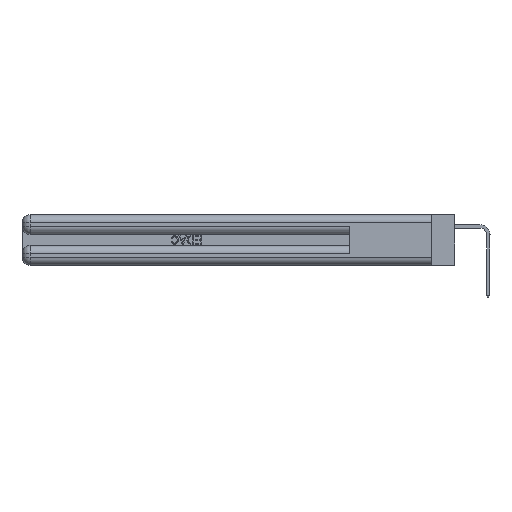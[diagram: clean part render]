
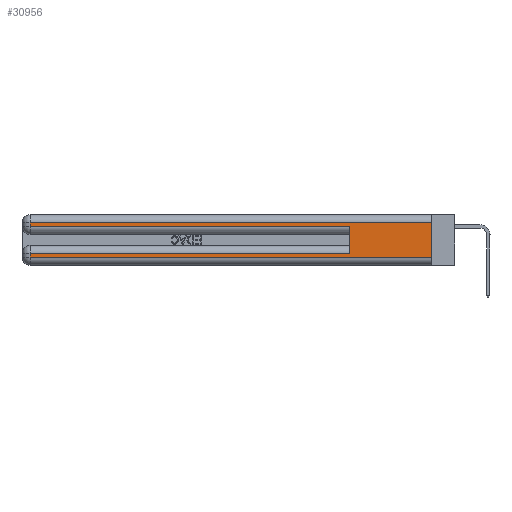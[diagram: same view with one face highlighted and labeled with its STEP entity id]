
A CAD part, left-side view. The second image highlights one B-rep face of the part: STEP entity #30956.
In plain terms, the highlighted planar face has unit normal (-1, 0, 0).
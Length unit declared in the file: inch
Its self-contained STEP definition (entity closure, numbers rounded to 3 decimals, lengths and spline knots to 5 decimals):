
#884 = CARTESIAN_POINT ( 'NONE',  ( 0., 2.94, 0.37 ) ) ;
#974 = VERTEX_POINT ( 'NONE', #17240 ) ;
#1247 = VECTOR ( 'NONE', #31002, 39.37008 ) ;
#1819 = VECTOR ( 'NONE', #13228, 39.37008 ) ;
#2746 = CARTESIAN_POINT ( 'NONE',  ( 0., 2.94, 0.37 ) ) ;
#3837 = VERTEX_POINT ( 'NONE', #28494 ) ;
#3931 = VERTEX_POINT ( 'NONE', #13141 ) ;
#4986 = CARTESIAN_POINT ( 'NONE',  ( 0., 0., 0.06 ) ) ;
#6003 = EDGE_CURVE ( 'NONE', #17276, #9255, #41050, .T. ) ;
#7483 = LINE ( 'NONE', #19568, #1819 ) ;
#8690 = EDGE_CURVE ( 'NONE', #9255, #3931, #18543, .T. ) ;
#9255 = VERTEX_POINT ( 'NONE', #15587 ) ;
#9530 = LINE ( 'NONE', #32223, #41440 ) ;
#9662 = VECTOR ( 'NONE', #33885, 39.37008 ) ;
#9823 = DIRECTION ( 'NONE',  ( 0., 0., -1. ) ) ;
#9946 = CARTESIAN_POINT ( 'NONE',  ( 0., 2.94, 0.31 ) ) ;
#10701 = CARTESIAN_POINT ( 'NONE',  ( 0., 0., 0.06 ) ) ;
#11762 = DIRECTION ( 'NONE',  ( 0., 1., 0. ) ) ;
#12237 = LINE ( 'NONE', #2746, #28236 ) ;
#13141 = CARTESIAN_POINT ( 'NONE',  ( 0., 0.6, 0.285 ) ) ;
#13228 = DIRECTION ( 'NONE',  ( 0., 0., -1. ) ) ;
#13327 = EDGE_CURVE ( 'NONE', #30325, #39252, #12237, .T. ) ;
#13684 = DIRECTION ( 'NONE',  ( 0., 1., 0. ) ) ;
#15205 = ORIENTED_EDGE ( 'NONE', *, *, #13327, .T. ) ;
#15587 = CARTESIAN_POINT ( 'NONE',  ( 0., 2.94, 0.285 ) ) ;
#15819 = LINE ( 'NONE', #29597, #32815 ) ;
#16313 = DIRECTION ( 'NONE',  ( 0., 0., 1. ) ) ;
#16717 = VECTOR ( 'NONE', #20326, 39.37008 ) ;
#16884 = ORIENTED_EDGE ( 'NONE', *, *, #39698, .T. ) ;
#17240 = CARTESIAN_POINT ( 'NONE',  ( 0., 0.6, 0.085 ) ) ;
#17276 = VERTEX_POINT ( 'NONE', #9946 ) ;
#18543 = LINE ( 'NONE', #27762, #1247 ) ;
#19428 = PLANE ( 'NONE',  #40757 ) ;
#19568 = CARTESIAN_POINT ( 'NONE',  ( 0., 0., 0.37 ) ) ;
#20326 = DIRECTION ( 'NONE',  ( 0., 0., -1. ) ) ;
#20951 = ORIENTED_EDGE ( 'NONE', *, *, #8690, .T. ) ;
#21142 = EDGE_CURVE ( 'NONE', #3837, #17276, #30302, .T. ) ;
#21417 = ORIENTED_EDGE ( 'NONE', *, *, #25348, .T. ) ;
#21894 = EDGE_LOOP ( 'NONE', ( #29300, #23803, #27504, #20951, #34060, #21417, #15205, #16884 ) ) ;
#22589 = CARTESIAN_POINT ( 'NONE',  ( 0., 0., 0.37 ) ) ;
#22780 = CARTESIAN_POINT ( 'NONE',  ( 0., 2.94, 0.085 ) ) ;
#23803 = ORIENTED_EDGE ( 'NONE', *, *, #21142, .T. ) ;
#25327 = DIRECTION ( 'NONE',  ( 0., 0., -1. ) ) ;
#25348 = EDGE_CURVE ( 'NONE', #974, #30325, #15819, .T. ) ;
#27504 = ORIENTED_EDGE ( 'NONE', *, *, #6003, .T. ) ;
#27688 = CARTESIAN_POINT ( 'NONE',  ( 0., 0., 0.31 ) ) ;
#27762 = CARTESIAN_POINT ( 'NONE',  ( 0., 0., 0.285 ) ) ;
#28236 = VECTOR ( 'NONE', #25327, 39.37008 ) ;
#28494 = CARTESIAN_POINT ( 'NONE',  ( 0., 0., 0.31 ) ) ;
#28708 = LINE ( 'NONE', #4986, #9662 ) ;
#29007 = DIRECTION ( 'NONE',  ( 1., 0., 0. ) ) ;
#29300 = ORIENTED_EDGE ( 'NONE', *, *, #35281, .F. ) ;
#29597 = CARTESIAN_POINT ( 'NONE',  ( 0., 0., 0.085 ) ) ;
#30302 = LINE ( 'NONE', #27688, #37712 ) ;
#30325 = VERTEX_POINT ( 'NONE', #22780 ) ;
#30956 = ADVANCED_FACE ( 'NONE', ( #39579 ), #19428, .F. ) ;
#31002 = DIRECTION ( 'NONE',  ( 0., -1., 0. ) ) ;
#32223 = CARTESIAN_POINT ( 'NONE',  ( 0., 0.6, 0.145 ) ) ;
#32815 = VECTOR ( 'NONE', #13684, 39.37008 ) ;
#33885 = DIRECTION ( 'NONE',  ( 0., -1., 0. ) ) ;
#34060 = ORIENTED_EDGE ( 'NONE', *, *, #35253, .F. ) ;
#35253 = EDGE_CURVE ( 'NONE', #974, #3931, #9530, .T. ) ;
#35281 = EDGE_CURVE ( 'NONE', #3837, #39596, #7483, .T. ) ;
#37712 = VECTOR ( 'NONE', #11762, 39.37008 ) ;
#39252 = VERTEX_POINT ( 'NONE', #40372 ) ;
#39579 = FACE_OUTER_BOUND ( 'NONE', #21894, .T. ) ;
#39596 = VERTEX_POINT ( 'NONE', #10701 ) ;
#39698 = EDGE_CURVE ( 'NONE', #39252, #39596, #28708, .T. ) ;
#40372 = CARTESIAN_POINT ( 'NONE',  ( 0., 2.94, 0.06 ) ) ;
#40757 = AXIS2_PLACEMENT_3D ( 'NONE', #22589, #29007, #9823 ) ;
#41050 = LINE ( 'NONE', #884, #16717 ) ;
#41440 = VECTOR ( 'NONE', #16313, 39.37008 ) ;
